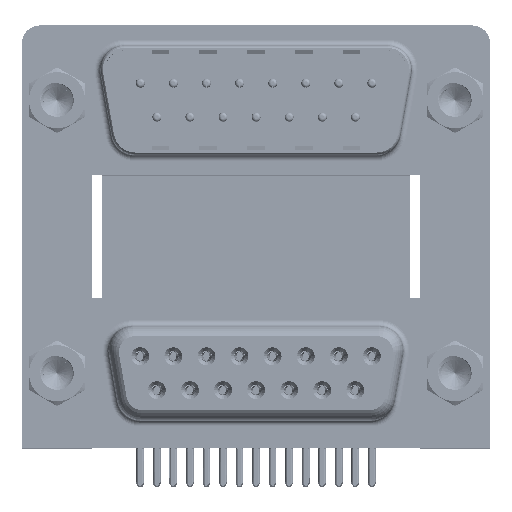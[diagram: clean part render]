
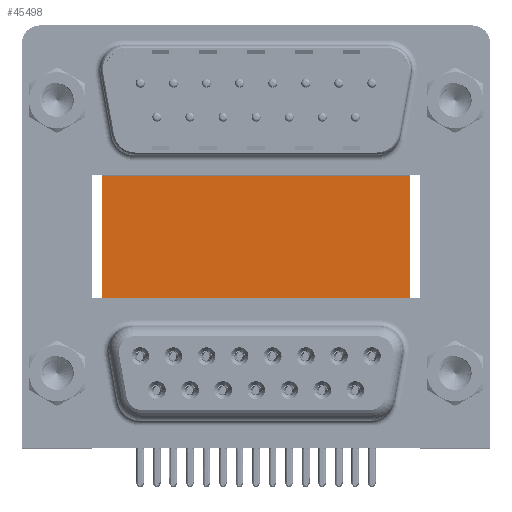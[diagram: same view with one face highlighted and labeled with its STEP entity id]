
A CAD part, top view. The second image highlights one B-rep face of the part: STEP entity #45498.
In plain terms, the highlighted planar face has unit normal (0, 0, 1).
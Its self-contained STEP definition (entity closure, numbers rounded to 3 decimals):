
#283 = CARTESIAN_POINT ( 'NONE',  ( 3.79, 16.585, -12. ) ) ;
#1478 = CARTESIAN_POINT ( 'NONE',  ( 3.79, 16.585, -12. ) ) ;
#1612 = CARTESIAN_POINT ( 'NONE',  ( 3.79, -3.735, -12. ) ) ;
#3499 = VECTOR ( 'NONE', #40095, 1000. ) ;
#9195 = EDGE_CURVE ( 'NONE', #46571, #31902, #35806, .T. ) ;
#9658 = CARTESIAN_POINT ( 'NONE',  ( 3.79, -3.735, -12. ) ) ;
#9771 = DIRECTION ( 'NONE',  ( -1., 0., 0. ) ) ;
#12118 = LINE ( 'NONE', #12625, #3499 ) ;
#12477 = ORIENTED_EDGE ( 'NONE', *, *, #26568, .T. ) ;
#12625 = CARTESIAN_POINT ( 'NONE',  ( 3.79, 16.585, -12. ) ) ;
#12699 = LINE ( 'NONE', #20239, #28137 ) ;
#13313 = LINE ( 'NONE', #9658, #41478 ) ;
#20239 = CARTESIAN_POINT ( 'NONE',  ( 29.58, 16.585, -12. ) ) ;
#20509 = ORIENTED_EDGE ( 'NONE', *, *, #23679, .F. ) ;
#23679 = EDGE_CURVE ( 'NONE', #27457, #46432, #12699, .T. ) ;
#24775 = ORIENTED_EDGE ( 'NONE', *, *, #9195, .T. ) ;
#25071 = PLANE ( 'NONE',  #32329 ) ;
#26568 = EDGE_CURVE ( 'NONE', #31902, #46432, #13313, .T. ) ;
#26840 = CARTESIAN_POINT ( 'NONE',  ( 29.58, 16.585, -12. ) ) ;
#27457 = VERTEX_POINT ( 'NONE', #26840 ) ;
#28137 = VECTOR ( 'NONE', #40175, 1000. ) ;
#31902 = VERTEX_POINT ( 'NONE', #1612 ) ;
#32329 = AXIS2_PLACEMENT_3D ( 'NONE', #1478, #33624, #9771 ) ;
#33624 = DIRECTION ( 'NONE',  ( 0., 0., -1. ) ) ;
#35420 = EDGE_LOOP ( 'NONE', ( #12477, #20509, #50173, #24775 ) ) ;
#35806 = LINE ( 'NONE', #283, #39176 ) ;
#39176 = VECTOR ( 'NONE', #47752, 1000. ) ;
#40095 = DIRECTION ( 'NONE',  ( 1., 0., 0. ) ) ;
#40175 = DIRECTION ( 'NONE',  ( 0., -1., 0. ) ) ;
#40277 = DIRECTION ( 'NONE',  ( 1., 0., 0. ) ) ;
#41306 = CARTESIAN_POINT ( 'NONE',  ( 29.58, -3.735, -12. ) ) ;
#41478 = VECTOR ( 'NONE', #40277, 1000. ) ;
#42846 = CARTESIAN_POINT ( 'NONE',  ( 3.79, 16.585, -12. ) ) ;
#45498 = ADVANCED_FACE ( 'NONE', ( #49209 ), #25071, .F. ) ;
#46432 = VERTEX_POINT ( 'NONE', #41306 ) ;
#46571 = VERTEX_POINT ( 'NONE', #42846 ) ;
#47752 = DIRECTION ( 'NONE',  ( 0., -1., 0. ) ) ;
#47997 = EDGE_CURVE ( 'NONE', #46571, #27457, #12118, .T. ) ;
#49209 = FACE_OUTER_BOUND ( 'NONE', #35420, .T. ) ;
#50173 = ORIENTED_EDGE ( 'NONE', *, *, #47997, .F. ) ;
